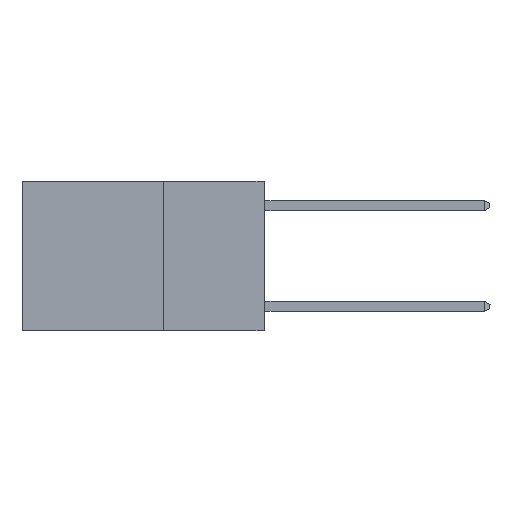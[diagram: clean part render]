
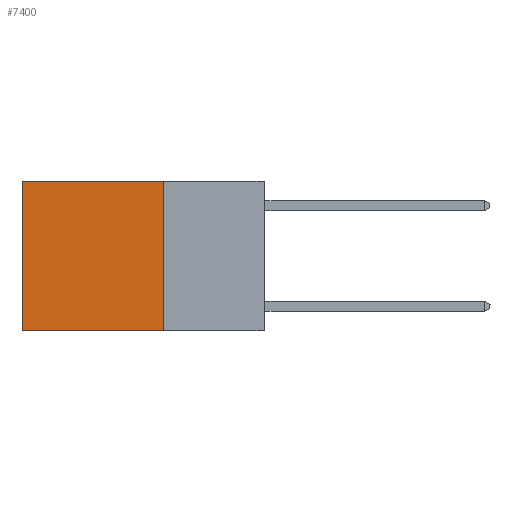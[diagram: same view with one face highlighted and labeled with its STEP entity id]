
A CAD part, left-side view. The second image highlights one B-rep face of the part: STEP entity #7400.
In plain terms, the highlighted planar face has unit normal (-1, 0, 0).
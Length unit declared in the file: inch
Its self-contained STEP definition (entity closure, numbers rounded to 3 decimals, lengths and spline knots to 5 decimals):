
#779 = DIRECTION ( 'NONE',  ( 0., 0., -1. ) ) ;
#1433 = EDGE_CURVE ( 'NONE', #17589, #10092, #2287, .T. ) ;
#1605 = DIRECTION ( 'NONE',  ( 1., 0., 0. ) ) ;
#2287 = LINE ( 'NONE', #10750, #6705 ) ;
#3387 = EDGE_LOOP ( 'NONE', ( #17096, #7426, #20731, #4546 ) ) ;
#4546 = ORIENTED_EDGE ( 'NONE', *, *, #14305, .T. ) ;
#5026 = VECTOR ( 'NONE', #8360, 39.37008 ) ;
#5075 = VERTEX_POINT ( 'NONE', #10902 ) ;
#6010 = LINE ( 'NONE', #13290, #9930 ) ;
#6673 = CARTESIAN_POINT ( 'NONE',  ( 0.2625, 0.6, 0. ) ) ;
#6705 = VECTOR ( 'NONE', #779, 39.37008 ) ;
#7400 = ADVANCED_FACE ( 'NONE', ( #13099 ), #8241, .F. ) ;
#7426 = ORIENTED_EDGE ( 'NONE', *, *, #19831, .F. ) ;
#8207 = LINE ( 'NONE', #10294, #16425 ) ;
#8241 = PLANE ( 'NONE',  #15393 ) ;
#8360 = DIRECTION ( 'NONE',  ( 0., 0., -1. ) ) ;
#9910 = CARTESIAN_POINT ( 'NONE',  ( 0.2625, 0.25, 0. ) ) ;
#9930 = VECTOR ( 'NONE', #14934, 39.37008 ) ;
#10092 = VERTEX_POINT ( 'NONE', #19480 ) ;
#10294 = CARTESIAN_POINT ( 'NONE',  ( 0.2625, 0.25, -0.37 ) ) ;
#10750 = CARTESIAN_POINT ( 'NONE',  ( 0.2625, 0.25, 0. ) ) ;
#10902 = CARTESIAN_POINT ( 'NONE',  ( 0.2625, 0.6, -0.37 ) ) ;
#13099 = FACE_OUTER_BOUND ( 'NONE', #3387, .T. ) ;
#13227 = DIRECTION ( 'NONE',  ( 0., 0., -1. ) ) ;
#13290 = CARTESIAN_POINT ( 'NONE',  ( 0.2625, 0.25, 0. ) ) ;
#13843 = LINE ( 'NONE', #6673, #5026 ) ;
#14305 = EDGE_CURVE ( 'NONE', #17589, #21386, #6010, .T. ) ;
#14934 = DIRECTION ( 'NONE',  ( 0., 1., 0. ) ) ;
#15393 = AXIS2_PLACEMENT_3D ( 'NONE', #9910, #1605, #13227 ) ;
#16425 = VECTOR ( 'NONE', #16943, 39.37008 ) ;
#16943 = DIRECTION ( 'NONE',  ( 0., 1., 0. ) ) ;
#17023 = CARTESIAN_POINT ( 'NONE',  ( 0.2625, 0.6, 0. ) ) ;
#17096 = ORIENTED_EDGE ( 'NONE', *, *, #20935, .T. ) ;
#17589 = VERTEX_POINT ( 'NONE', #19940 ) ;
#19480 = CARTESIAN_POINT ( 'NONE',  ( 0.2625, 0.25, -0.37 ) ) ;
#19831 = EDGE_CURVE ( 'NONE', #10092, #5075, #8207, .T. ) ;
#19940 = CARTESIAN_POINT ( 'NONE',  ( 0.2625, 0.25, 0. ) ) ;
#20731 = ORIENTED_EDGE ( 'NONE', *, *, #1433, .F. ) ;
#20935 = EDGE_CURVE ( 'NONE', #21386, #5075, #13843, .T. ) ;
#21386 = VERTEX_POINT ( 'NONE', #17023 ) ;
